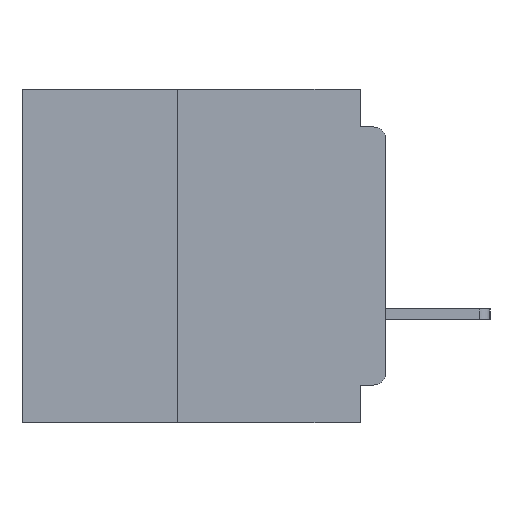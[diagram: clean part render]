
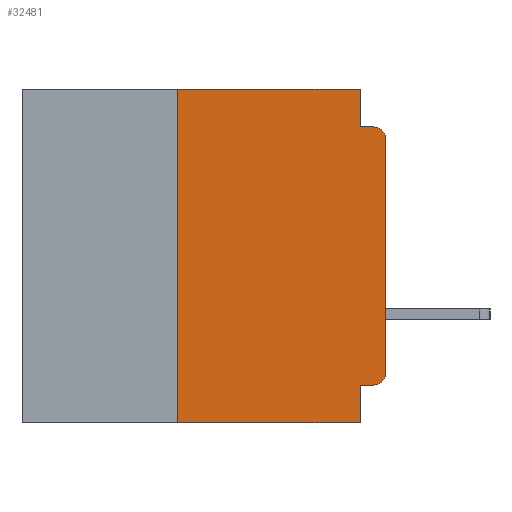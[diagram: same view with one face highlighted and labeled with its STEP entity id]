
A CAD part, left-side view. The second image highlights one B-rep face of the part: STEP entity #32481.
In plain terms, the highlighted planar face has unit normal (-1, 0, 0).
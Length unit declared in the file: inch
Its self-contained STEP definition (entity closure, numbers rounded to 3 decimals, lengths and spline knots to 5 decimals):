
#402 = CARTESIAN_POINT ( 'NONE',  ( 0., 0.25, -0.4 ) ) ;
#1037 = EDGE_CURVE ( 'NONE', #57977, #51216, #36298, .T. ) ;
#2374 = LINE ( 'NONE', #6177, #54368 ) ;
#2471 = AXIS2_PLACEMENT_3D ( 'NONE', #49280, #20016, #54154 ) ;
#3213 = FACE_OUTER_BOUND ( 'NONE', #27929, .T. ) ;
#3438 = DIRECTION ( 'NONE',  ( 1., 0., 0. ) ) ;
#4365 = CARTESIAN_POINT ( 'NONE',  ( 0., 0., -0.06 ) ) ;
#4383 = DIRECTION ( 'NONE',  ( 0., 0., -1. ) ) ;
#4761 = ORIENTED_EDGE ( 'NONE', *, *, #36521, .T. ) ;
#4976 = AXIS2_PLACEMENT_3D ( 'NONE', #52903, #23652, #57747 ) ;
#5645 = CARTESIAN_POINT ( 'NONE',  ( 0., 0., -0.34 ) ) ;
#5985 = VECTOR ( 'NONE', #13492, 39.37008 ) ;
#6007 = CARTESIAN_POINT ( 'NONE',  ( 0., 0.015, -0.045 ) ) ;
#6043 = EDGE_CURVE ( 'NONE', #54245, #28536, #27742, .T. ) ;
#6177 = CARTESIAN_POINT ( 'NONE',  ( 0., 0., 0. ) ) ;
#7284 = EDGE_CURVE ( 'NONE', #28536, #59937, #2374, .T. ) ;
#9054 = LINE ( 'NONE', #46624, #22051 ) ;
#11569 = CARTESIAN_POINT ( 'NONE',  ( 0., 0.031, -0.045 ) ) ;
#12469 = DIRECTION ( 'NONE',  ( 0., -1., 0. ) ) ;
#13492 = DIRECTION ( 'NONE',  ( 0., 0., 1. ) ) ;
#13677 = EDGE_CURVE ( 'NONE', #60708, #51216, #46058, .T. ) ;
#16056 = ORIENTED_EDGE ( 'NONE', *, *, #7284, .T. ) ;
#17243 = VERTEX_POINT ( 'NONE', #11569 ) ;
#17595 = VERTEX_POINT ( 'NONE', #43507 ) ;
#19019 = EDGE_CURVE ( 'NONE', #17595, #49269, #33974, .T. ) ;
#20016 = DIRECTION ( 'NONE',  ( -1., 0., 0. ) ) ;
#20945 = EDGE_CURVE ( 'NONE', #17243, #35683, #9054, .T. ) ;
#22051 = VECTOR ( 'NONE', #12469, 39.37008 ) ;
#23652 = DIRECTION ( 'NONE',  ( -1., 0., 0. ) ) ;
#25904 = CARTESIAN_POINT ( 'NONE',  ( 0., 0.031, -0.4 ) ) ;
#27300 = CARTESIAN_POINT ( 'NONE',  ( 0., 0., -0.355 ) ) ;
#27742 = CIRCLE ( 'NONE', #2471, 0.015 ) ;
#27929 = EDGE_LOOP ( 'NONE', ( #16056, #4761, #56235, #57152, #55458, #48317, #61656, #58311, #61307, #34595 ) ) ;
#28536 = VERTEX_POINT ( 'NONE', #5645 ) ;
#28773 = CARTESIAN_POINT ( 'NONE',  ( 0., 0.031, -0.4 ) ) ;
#30351 = CIRCLE ( 'NONE', #4976, 0.015 ) ;
#30801 = DIRECTION ( 'NONE',  ( 0., -1., 0. ) ) ;
#32481 = ADVANCED_FACE ( 'NONE', ( #3213 ), #33003, .F. ) ;
#33003 = PLANE ( 'NONE',  #62392 ) ;
#33113 = VECTOR ( 'NONE', #50861, 39.37008 ) ;
#33974 = LINE ( 'NONE', #59918, #46948 ) ;
#34595 = ORIENTED_EDGE ( 'NONE', *, *, #6043, .T. ) ;
#35683 = VERTEX_POINT ( 'NONE', #6007 ) ;
#36298 = LINE ( 'NONE', #28773, #60628 ) ;
#36521 = EDGE_CURVE ( 'NONE', #59937, #35683, #30351, .T. ) ;
#36758 = LINE ( 'NONE', #27300, #49780 ) ;
#37856 = DIRECTION ( 'NONE',  ( 0., 0., -1. ) ) ;
#38956 = CARTESIAN_POINT ( 'NONE',  ( 0., 0.015, -0.355 ) ) ;
#40335 = DIRECTION ( 'NONE',  ( 0., 0., 1. ) ) ;
#43507 = CARTESIAN_POINT ( 'NONE',  ( 0., 0.25, 0. ) ) ;
#44011 = VECTOR ( 'NONE', #47835, 39.37008 ) ;
#46058 = LINE ( 'NONE', #55715, #33113 ) ;
#46624 = CARTESIAN_POINT ( 'NONE',  ( 0., 0., -0.045 ) ) ;
#46948 = VECTOR ( 'NONE', #30801, 39.37008 ) ;
#47618 = CARTESIAN_POINT ( 'NONE',  ( 0., 0.25, -0.4 ) ) ;
#47835 = DIRECTION ( 'NONE',  ( 0., 0., -1. ) ) ;
#48317 = ORIENTED_EDGE ( 'NONE', *, *, #51517, .F. ) ;
#49269 = VERTEX_POINT ( 'NONE', #59332 ) ;
#49280 = CARTESIAN_POINT ( 'NONE',  ( 0., 0.015, -0.34 ) ) ;
#49780 = VECTOR ( 'NONE', #56480, 39.37008 ) ;
#50131 = EDGE_CURVE ( 'NONE', #54245, #57977, #36758, .T. ) ;
#50861 = DIRECTION ( 'NONE',  ( 0., -1., 0. ) ) ;
#51216 = VERTEX_POINT ( 'NONE', #25904 ) ;
#51517 = EDGE_CURVE ( 'NONE', #60708, #17595, #57902, .T. ) ;
#52903 = CARTESIAN_POINT ( 'NONE',  ( 0., 0.015, -0.06 ) ) ;
#54154 = DIRECTION ( 'NONE',  ( 0., 0., -1. ) ) ;
#54245 = VERTEX_POINT ( 'NONE', #38956 ) ;
#54368 = VECTOR ( 'NONE', #40335, 39.37008 ) ;
#55458 = ORIENTED_EDGE ( 'NONE', *, *, #19019, .F. ) ;
#55715 = CARTESIAN_POINT ( 'NONE',  ( 0., 0.437, -0.4 ) ) ;
#56235 = ORIENTED_EDGE ( 'NONE', *, *, #20945, .F. ) ;
#56480 = DIRECTION ( 'NONE',  ( 0., 1., 0. ) ) ;
#57152 = ORIENTED_EDGE ( 'NONE', *, *, #57992, .F. ) ;
#57262 = CARTESIAN_POINT ( 'NONE',  ( 0., 0.437, 0. ) ) ;
#57590 = CARTESIAN_POINT ( 'NONE',  ( 0., 0.031, 0. ) ) ;
#57747 = DIRECTION ( 'NONE',  ( 0., 0., -1. ) ) ;
#57902 = LINE ( 'NONE', #47618, #5985 ) ;
#57977 = VERTEX_POINT ( 'NONE', #62191 ) ;
#57992 = EDGE_CURVE ( 'NONE', #49269, #17243, #58481, .T. ) ;
#58311 = ORIENTED_EDGE ( 'NONE', *, *, #1037, .F. ) ;
#58481 = LINE ( 'NONE', #57590, #44011 ) ;
#59332 = CARTESIAN_POINT ( 'NONE',  ( 0., 0.031, 0. ) ) ;
#59918 = CARTESIAN_POINT ( 'NONE',  ( 0., 0.437, 0. ) ) ;
#59937 = VERTEX_POINT ( 'NONE', #4365 ) ;
#60628 = VECTOR ( 'NONE', #4383, 39.37008 ) ;
#60708 = VERTEX_POINT ( 'NONE', #402 ) ;
#61307 = ORIENTED_EDGE ( 'NONE', *, *, #50131, .F. ) ;
#61656 = ORIENTED_EDGE ( 'NONE', *, *, #13677, .T. ) ;
#62191 = CARTESIAN_POINT ( 'NONE',  ( 0., 0.031, -0.355 ) ) ;
#62392 = AXIS2_PLACEMENT_3D ( 'NONE', #57262, #3438, #37856 ) ;
